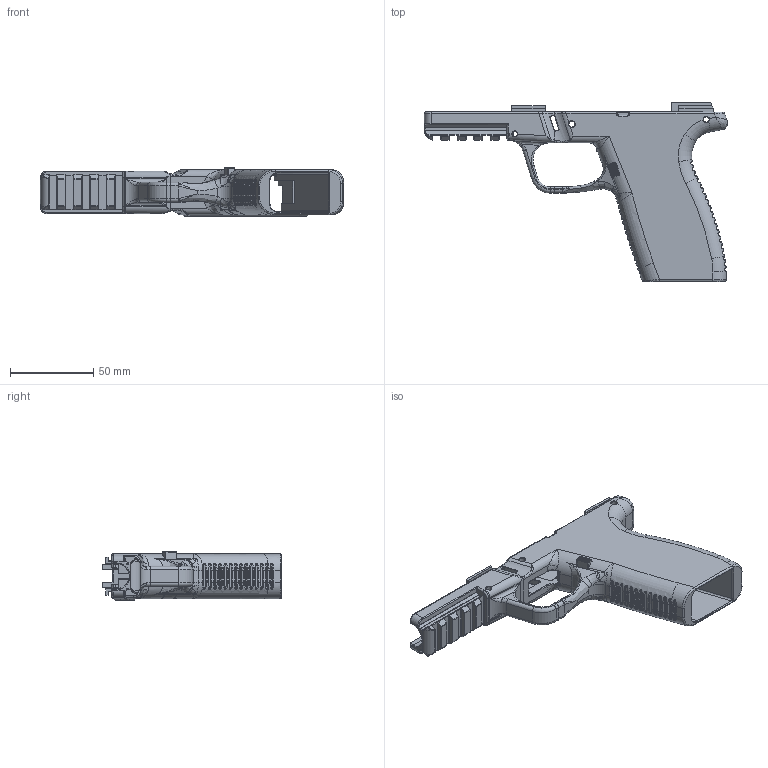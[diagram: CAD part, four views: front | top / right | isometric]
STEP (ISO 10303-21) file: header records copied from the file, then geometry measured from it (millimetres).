
FILE_DESCRIPTION(/* description */ (''),/* implementation_level */ '2;1');
FILE_NAME(/* name */ 'SW9 Glock Edition.step',/* time_stamp */ '2021-10-26T17:42:32-04:00',/* author */ (''),/* organization */ (''),/* preprocessor_version */ 'ST-DEVELOPER v18.1',/* originating_system */ 'Autodesk Translation Framework v10.10.0.1391',/* authorisation */ '');
FILE_SCHEMA (('AUTOMOTIVE_DESIGN { 1 0 10303 214 3 1 1 }'));
Products named in the file (5): SW9 Glock Edition; Rail; Mag Catch v2; SW9 Module; Rail Spec
Assembly tree (4 placements, depth 2):
  SW9 Glock Edition
    Rail
    Mag Catch v2
    SW9 Module
    Rail Spec
Bounding box: 181.88 x 107.38 x 29.37 mm (x, y, z)
Volume: 90610.7 mm3; surface area: 54118.5 mm2
Topology: 7 solids, 7 shells, 1957 faces, 4875 edges, 2840 vertices
Faces by surface type: cylinder 657, bspline 654, plane 407, torus 182, sphere 37, cone 20
Full cylindrical faces by diameter (mm): 3.175 x3, 3.3 x5, 3.6 x2
Entity records: 80814 total; most frequent: CARTESIAN_POINT 36738, ORIENTED_EDGE 9588, DIRECTION 8820, EDGE_CURVE 4794, AXIS2_PLACEMENT_3D 3560, VERTEX_POINT 2838, EDGE_LOOP 1974, FACE_OUTER_BOUND 1957
